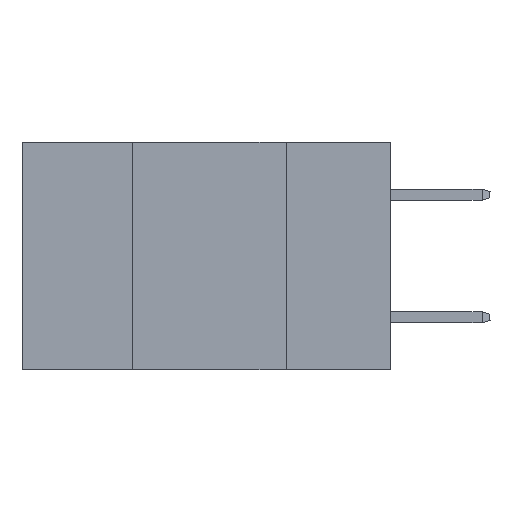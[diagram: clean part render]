
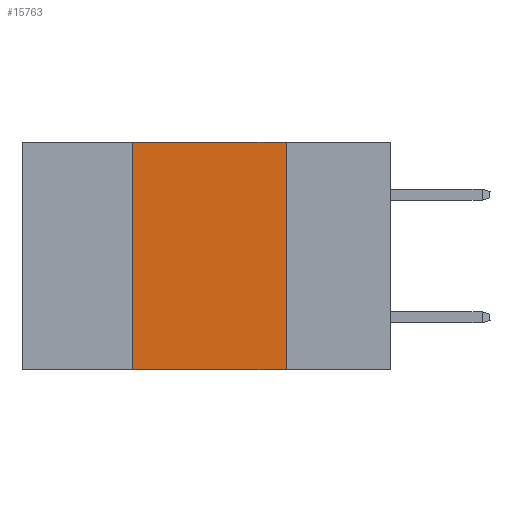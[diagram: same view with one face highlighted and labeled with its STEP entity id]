
A CAD part, left-side view. The second image highlights one B-rep face of the part: STEP entity #15763.
In plain terms, the highlighted planar face has unit normal (-1, 0, 0).
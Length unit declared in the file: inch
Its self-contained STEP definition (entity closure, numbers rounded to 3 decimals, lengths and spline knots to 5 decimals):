
#2564 = CARTESIAN_POINT ( 'NONE',  ( 0., 0.17, 0. ) ) ;
#4325 = VECTOR ( 'NONE', #21506, 39.37008 ) ;
#4704 = VECTOR ( 'NONE', #32422, 39.37008 ) ;
#5586 = CARTESIAN_POINT ( 'NONE',  ( 0., 0.42, -0.37 ) ) ;
#7731 = DIRECTION ( 'NONE',  ( 0., -1., 0. ) ) ;
#8084 = VECTOR ( 'NONE', #32435, 39.37008 ) ;
#8484 = EDGE_LOOP ( 'NONE', ( #22444, #29516, #32823, #31074 ) ) ;
#9196 = EDGE_CURVE ( 'NONE', #27880, #19094, #16125, .T. ) ;
#9558 = DIRECTION ( 'NONE',  ( 0., 0., -1. ) ) ;
#12289 = CARTESIAN_POINT ( 'NONE',  ( 0., 0.6, 0. ) ) ;
#13185 = CARTESIAN_POINT ( 'NONE',  ( 0., 0.6, -0.37 ) ) ;
#13417 = CARTESIAN_POINT ( 'NONE',  ( 0., 0.6, 0. ) ) ;
#14103 = CARTESIAN_POINT ( 'NONE',  ( 0., 0.42, 0. ) ) ;
#15728 = LINE ( 'NONE', #2564, #4325 ) ;
#15763 = ADVANCED_FACE ( 'NONE', ( #16352 ), #28726, .F. ) ;
#16125 = LINE ( 'NONE', #13417, #8084 ) ;
#16352 = FACE_OUTER_BOUND ( 'NONE', #8484, .T. ) ;
#16855 = AXIS2_PLACEMENT_3D ( 'NONE', #12289, #17940, #9558 ) ;
#17743 = EDGE_CURVE ( 'NONE', #19272, #34875, #18923, .T. ) ;
#17940 = DIRECTION ( 'NONE',  ( 1., 0., 0. ) ) ;
#18923 = LINE ( 'NONE', #13185, #26540 ) ;
#19094 = VERTEX_POINT ( 'NONE', #24175 ) ;
#19272 = VERTEX_POINT ( 'NONE', #5586 ) ;
#21506 = DIRECTION ( 'NONE',  ( 0., 0., -1. ) ) ;
#22444 = ORIENTED_EDGE ( 'NONE', *, *, #32059, .F. ) ;
#24175 = CARTESIAN_POINT ( 'NONE',  ( 0., 0.17, 0. ) ) ;
#24398 = CARTESIAN_POINT ( 'NONE',  ( 0., 0.42, 0. ) ) ;
#25623 = CARTESIAN_POINT ( 'NONE',  ( 0., 0.17, -0.37 ) ) ;
#26540 = VECTOR ( 'NONE', #7731, 39.37008 ) ;
#27880 = VERTEX_POINT ( 'NONE', #14103 ) ;
#28726 = PLANE ( 'NONE',  #16855 ) ;
#29516 = ORIENTED_EDGE ( 'NONE', *, *, #9196, .F. ) ;
#30500 = LINE ( 'NONE', #24398, #4704 ) ;
#31074 = ORIENTED_EDGE ( 'NONE', *, *, #17743, .T. ) ;
#32059 = EDGE_CURVE ( 'NONE', #19094, #34875, #15728, .T. ) ;
#32422 = DIRECTION ( 'NONE',  ( 0., 0., 1. ) ) ;
#32435 = DIRECTION ( 'NONE',  ( 0., -1., 0. ) ) ;
#32823 = ORIENTED_EDGE ( 'NONE', *, *, #32828, .F. ) ;
#32828 = EDGE_CURVE ( 'NONE', #19272, #27880, #30500, .T. ) ;
#34875 = VERTEX_POINT ( 'NONE', #25623 ) ;
